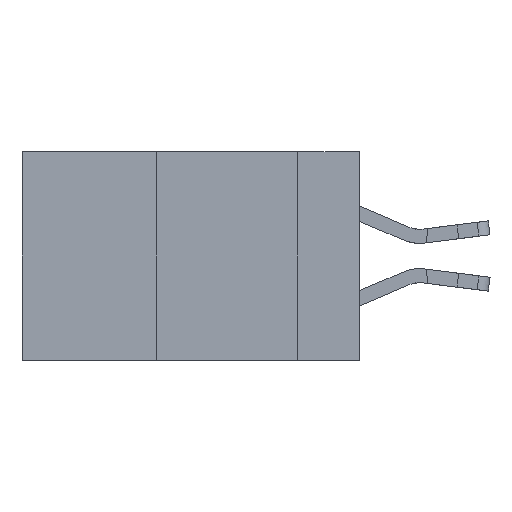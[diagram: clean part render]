
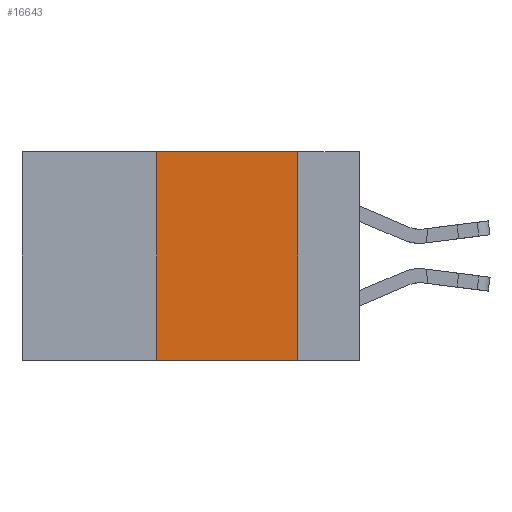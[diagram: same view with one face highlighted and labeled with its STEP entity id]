
A CAD part, left-side view. The second image highlights one B-rep face of the part: STEP entity #16643.
In plain terms, the highlighted planar face has unit normal (-1, 0, 0).
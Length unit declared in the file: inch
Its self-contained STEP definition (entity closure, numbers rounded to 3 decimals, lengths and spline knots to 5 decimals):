
#1722 = CARTESIAN_POINT ( 'NONE',  ( 0., 0.11, 0. ) ) ;
#2728 = LINE ( 'NONE', #17338, #12444 ) ;
#2767 = DIRECTION ( 'NONE',  ( 1., 0., 0. ) ) ;
#3913 = CARTESIAN_POINT ( 'NONE',  ( 0., 0.11, -0.37 ) ) ;
#4559 = CARTESIAN_POINT ( 'NONE',  ( 0., 0.36, 0. ) ) ;
#4898 = DIRECTION ( 'NONE',  ( 0., 0., -1. ) ) ;
#7395 = EDGE_CURVE ( 'NONE', #14766, #15669, #25267, .T. ) ;
#8439 = EDGE_CURVE ( 'NONE', #19531, #28297, #2728, .T. ) ;
#8997 = PLANE ( 'NONE',  #16280 ) ;
#9100 = DIRECTION ( 'NONE',  ( 0., -1., 0. ) ) ;
#9114 = FACE_OUTER_BOUND ( 'NONE', #15026, .T. ) ;
#9485 = DIRECTION ( 'NONE',  ( 0., 0., 1. ) ) ;
#9521 = VECTOR ( 'NONE', #9100, 39.37008 ) ;
#10857 = DIRECTION ( 'NONE',  ( 0., -1., 0. ) ) ;
#11696 = CARTESIAN_POINT ( 'NONE',  ( 0., 0.6, 0. ) ) ;
#11820 = ORIENTED_EDGE ( 'NONE', *, *, #25750, .F. ) ;
#11973 = CARTESIAN_POINT ( 'NONE',  ( 0., 0.36, 0. ) ) ;
#12247 = VECTOR ( 'NONE', #15126, 39.37008 ) ;
#12444 = VECTOR ( 'NONE', #10857, 39.37008 ) ;
#13606 = VECTOR ( 'NONE', #9485, 39.37008 ) ;
#14766 = VERTEX_POINT ( 'NONE', #4559 ) ;
#14830 = CARTESIAN_POINT ( 'NONE',  ( 0., 0.11, 0. ) ) ;
#15026 = EDGE_LOOP ( 'NONE', ( #11820, #26642, #23878, #21125 ) ) ;
#15126 = DIRECTION ( 'NONE',  ( 0., 0., -1. ) ) ;
#15669 = VERTEX_POINT ( 'NONE', #14830 ) ;
#15911 = CARTESIAN_POINT ( 'NONE',  ( 0., 0.6, 0. ) ) ;
#16280 = AXIS2_PLACEMENT_3D ( 'NONE', #15911, #2767, #4898 ) ;
#16643 = ADVANCED_FACE ( 'NONE', ( #9114 ), #8997, .F. ) ;
#16815 = EDGE_CURVE ( 'NONE', #19531, #14766, #25870, .T. ) ;
#16994 = CARTESIAN_POINT ( 'NONE',  ( 0., 0.36, -0.37 ) ) ;
#17338 = CARTESIAN_POINT ( 'NONE',  ( 0., 0.6, -0.37 ) ) ;
#19531 = VERTEX_POINT ( 'NONE', #16994 ) ;
#21125 = ORIENTED_EDGE ( 'NONE', *, *, #8439, .T. ) ;
#23155 = LINE ( 'NONE', #1722, #12247 ) ;
#23878 = ORIENTED_EDGE ( 'NONE', *, *, #16815, .F. ) ;
#25267 = LINE ( 'NONE', #11696, #9521 ) ;
#25750 = EDGE_CURVE ( 'NONE', #15669, #28297, #23155, .T. ) ;
#25870 = LINE ( 'NONE', #11973, #13606 ) ;
#26642 = ORIENTED_EDGE ( 'NONE', *, *, #7395, .F. ) ;
#28297 = VERTEX_POINT ( 'NONE', #3913 ) ;
